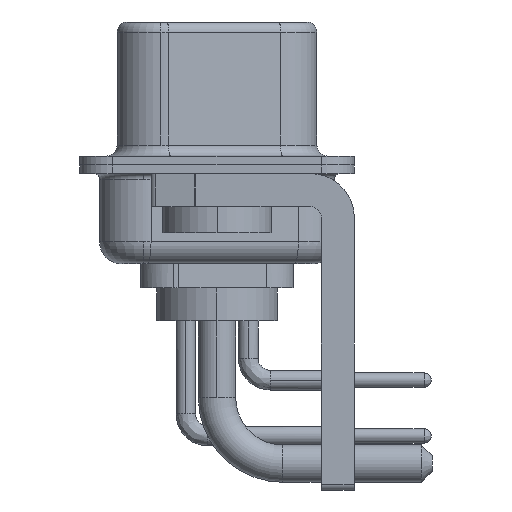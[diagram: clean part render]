
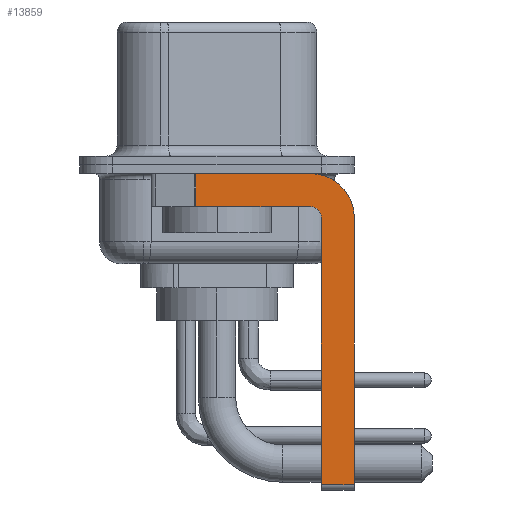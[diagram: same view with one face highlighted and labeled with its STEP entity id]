
A CAD part, left-side view. The second image highlights one B-rep face of the part: STEP entity #13859.
In plain terms, the highlighted planar face has unit normal (-1, 0, 0).
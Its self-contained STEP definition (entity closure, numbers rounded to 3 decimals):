
#123 = DIRECTION ( 'NONE',  ( 0., 0., -1. ) ) ;
#358 = VECTOR ( 'NONE', #14338, 1000. ) ;
#460 = DIRECTION ( 'NONE',  ( 1., 0., 0. ) ) ;
#1056 = DIRECTION ( 'NONE',  ( 0., 0., -1. ) ) ;
#2129 = LINE ( 'NONE', #23731, #16427 ) ;
#2443 = CARTESIAN_POINT ( 'NONE',  ( -2.9, 0.978, -1.9 ) ) ;
#2505 = DIRECTION ( 'NONE',  ( 0., 1., 0. ) ) ;
#3712 = AXIS2_PLACEMENT_3D ( 'NONE', #12067, #12191, #123 ) ;
#4404 = CARTESIAN_POINT ( 'NONE',  ( -2.9, -4.25, -0.4 ) ) ;
#4756 = VERTEX_POINT ( 'NONE', #5860 ) ;
#4798 = CARTESIAN_POINT ( 'NONE',  ( -2.9, -6.25, -14.55 ) ) ;
#5412 = CARTESIAN_POINT ( 'NONE',  ( -2.9, 3., -0.4 ) ) ;
#5631 = CARTESIAN_POINT ( 'NONE',  ( -2.9, 0.978, -1.9 ) ) ;
#5817 = EDGE_CURVE ( 'NONE', #6626, #10051, #16045, .T. ) ;
#5860 = CARTESIAN_POINT ( 'NONE',  ( -2.9, -4.75, -2.4 ) ) ;
#6042 = CARTESIAN_POINT ( 'NONE',  ( -2.9, -4.25, -14.55 ) ) ;
#6346 = ORIENTED_EDGE ( 'NONE', *, *, #20961, .T. ) ;
#6387 = FACE_OUTER_BOUND ( 'NONE', #7943, .T. ) ;
#6626 = VERTEX_POINT ( 'NONE', #4404 ) ;
#7839 = EDGE_CURVE ( 'NONE', #18094, #17170, #2129, .T. ) ;
#7943 = EDGE_LOOP ( 'NONE', ( #8437, #14073, #16397, #12493, #9856, #6346, #11099, #12019 ) ) ;
#8437 = ORIENTED_EDGE ( 'NONE', *, *, #11547, .F. ) ;
#8895 = VERTEX_POINT ( 'NONE', #17066 ) ;
#9094 = CIRCLE ( 'NONE', #22249, 0.5 ) ;
#9255 = EDGE_CURVE ( 'NONE', #4756, #18094, #9094, .T. ) ;
#9856 = ORIENTED_EDGE ( 'NONE', *, *, #21537, .F. ) ;
#10051 = VERTEX_POINT ( 'NONE', #11964 ) ;
#10122 = VERTEX_POINT ( 'NONE', #24326 ) ;
#10369 = CARTESIAN_POINT ( 'NONE',  ( -2.9, -4.25, -2.4 ) ) ;
#10831 = EDGE_CURVE ( 'NONE', #8895, #17170, #13200, .T. ) ;
#11099 = ORIENTED_EDGE ( 'NONE', *, *, #22103, .F. ) ;
#11547 = EDGE_CURVE ( 'NONE', #8895, #6626, #23136, .T. ) ;
#11895 = PLANE ( 'NONE',  #22366 ) ;
#11964 = CARTESIAN_POINT ( 'NONE',  ( -2.9, -6.25, -2.4 ) ) ;
#12019 = ORIENTED_EDGE ( 'NONE', *, *, #5817, .F. ) ;
#12067 = CARTESIAN_POINT ( 'NONE',  ( -2.9, -4.25, -2.4 ) ) ;
#12191 = DIRECTION ( 'NONE',  ( 1., 0., 0. ) ) ;
#12493 = ORIENTED_EDGE ( 'NONE', *, *, #9255, .F. ) ;
#13200 = LINE ( 'NONE', #5631, #25111 ) ;
#13238 = DIRECTION ( 'NONE',  ( 0., -1., 0. ) ) ;
#13326 = DIRECTION ( 'NONE',  ( 0., 0., -1. ) ) ;
#13854 = DIRECTION ( 'NONE',  ( 0., -1., 0. ) ) ;
#13859 = ADVANCED_FACE ( 'NONE', ( #6387 ), #11895, .F. ) ;
#14073 = ORIENTED_EDGE ( 'NONE', *, *, #10831, .T. ) ;
#14338 = DIRECTION ( 'NONE',  ( 0., 0., 1. ) ) ;
#14479 = CARTESIAN_POINT ( 'NONE',  ( -2.9, -4.25, -2.4 ) ) ;
#14880 = VECTOR ( 'NONE', #13238, 1000. ) ;
#16010 = LINE ( 'NONE', #18080, #358 ) ;
#16045 = CIRCLE ( 'NONE', #3712, 2. ) ;
#16160 = CARTESIAN_POINT ( 'NONE',  ( -2.9, -4.25, -1.9 ) ) ;
#16397 = ORIENTED_EDGE ( 'NONE', *, *, #7839, .F. ) ;
#16427 = VECTOR ( 'NONE', #2505, 1000. ) ;
#16628 = CARTESIAN_POINT ( 'NONE',  ( -2.9, -6.25, -2.4 ) ) ;
#17066 = CARTESIAN_POINT ( 'NONE',  ( -2.9, 0.978, -0.4 ) ) ;
#17170 = VERTEX_POINT ( 'NONE', #2443 ) ;
#18080 = CARTESIAN_POINT ( 'NONE',  ( -2.9, -4.75, -14.8 ) ) ;
#18094 = VERTEX_POINT ( 'NONE', #16160 ) ;
#18226 = DIRECTION ( 'NONE',  ( 0., 0., 1. ) ) ;
#18693 = LINE ( 'NONE', #16628, #18858 ) ;
#18858 = VECTOR ( 'NONE', #1056, 1000. ) ;
#19234 = VECTOR ( 'NONE', #13854, 1000. ) ;
#20268 = DIRECTION ( 'NONE',  ( -1., 0., 0. ) ) ;
#20961 = EDGE_CURVE ( 'NONE', #10122, #24457, #23634, .T. ) ;
#21537 = EDGE_CURVE ( 'NONE', #10122, #4756, #16010, .T. ) ;
#21811 = DIRECTION ( 'NONE',  ( 0., 0., -1. ) ) ;
#22103 = EDGE_CURVE ( 'NONE', #10051, #24457, #18693, .T. ) ;
#22249 = AXIS2_PLACEMENT_3D ( 'NONE', #10369, #20268, #18226 ) ;
#22366 = AXIS2_PLACEMENT_3D ( 'NONE', #14479, #460, #21811 ) ;
#23136 = LINE ( 'NONE', #5412, #14880 ) ;
#23634 = LINE ( 'NONE', #6042, #19234 ) ;
#23731 = CARTESIAN_POINT ( 'NONE',  ( -2.9, -4.25, -1.9 ) ) ;
#24326 = CARTESIAN_POINT ( 'NONE',  ( -2.9, -4.75, -14.55 ) ) ;
#24457 = VERTEX_POINT ( 'NONE', #4798 ) ;
#25111 = VECTOR ( 'NONE', #13326, 1000. ) ;
